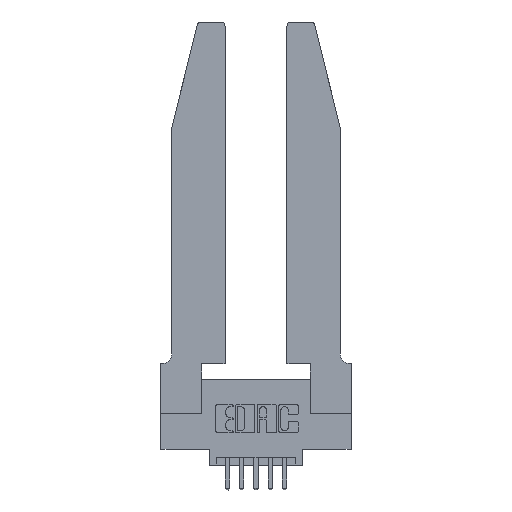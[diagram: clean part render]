
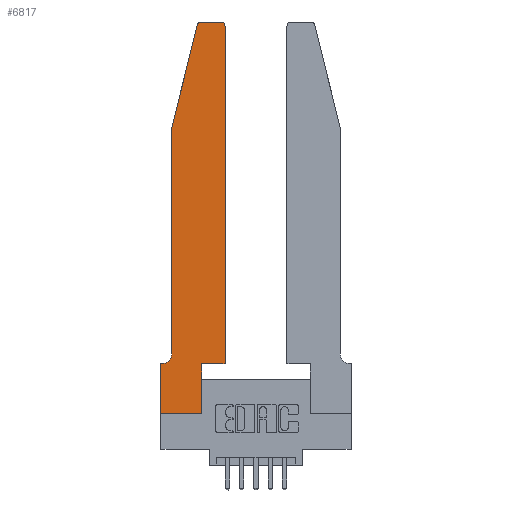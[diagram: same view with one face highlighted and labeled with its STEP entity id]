
A CAD part, top view. The second image highlights one B-rep face of the part: STEP entity #6817.
In plain terms, the highlighted planar face has unit normal (0, 0, 1).
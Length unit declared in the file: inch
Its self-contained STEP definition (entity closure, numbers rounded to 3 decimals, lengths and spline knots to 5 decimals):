
#37 = DIRECTION ( 'NONE',  ( -1., 0., 0. ) ) ;
#279 = CARTESIAN_POINT ( 'NONE',  ( 0., 0., 0.37 ) ) ;
#333 = FACE_OUTER_BOUND ( 'NONE', #13495, .T. ) ;
#451 = CARTESIAN_POINT ( 'NONE',  ( 0.25487, 2.72718, 0.37 ) ) ;
#506 = CIRCLE ( 'NONE', #3302, 0.03 ) ;
#507 = DIRECTION ( 'NONE',  ( 1., 0., 0. ) ) ;
#512 = VECTOR ( 'NONE', #12352, 39.37008 ) ;
#652 = VERTEX_POINT ( 'NONE', #10026 ) ;
#686 = CARTESIAN_POINT ( 'NONE',  ( 0.284, 2.75, 0.37 ) ) ;
#1162 = DIRECTION ( 'NONE',  ( 1., 0., 0. ) ) ;
#1601 = VECTOR ( 'NONE', #37, 39.37008 ) ;
#1735 = CARTESIAN_POINT ( 'NONE',  ( 0.4205, 2.75, 0.37 ) ) ;
#1758 = ORIENTED_EDGE ( 'NONE', *, *, #10402, .T. ) ;
#1817 = CARTESIAN_POINT ( 'NONE',  ( 0., 0.35, 0.37 ) ) ;
#2242 = VECTOR ( 'NONE', #5406, 39.37008 ) ;
#2355 = EDGE_CURVE ( 'NONE', #13267, #9905, #3625, .T. ) ;
#2409 = LINE ( 'NONE', #9857, #2242 ) ;
#2546 = CARTESIAN_POINT ( 'NONE',  ( 0.4505, 2.72, 0.37 ) ) ;
#2553 = LINE ( 'NONE', #13934, #6417 ) ;
#3101 = VECTOR ( 'NONE', #4909, 39.37008 ) ;
#3121 = CARTESIAN_POINT ( 'NONE',  ( 0.0755, 2., 0.37 ) ) ;
#3213 = CARTESIAN_POINT ( 'NONE',  ( 0.2605, 2.75, 0.37 ) ) ;
#3248 = VECTOR ( 'NONE', #7349, 39.37008 ) ;
#3302 = AXIS2_PLACEMENT_3D ( 'NONE', #6360, #9641, #8470 ) ;
#3325 = VERTEX_POINT ( 'NONE', #3121 ) ;
#3347 = DIRECTION ( 'NONE',  ( 0., 0., -1. ) ) ;
#3625 = CIRCLE ( 'NONE', #7901, 0.03 ) ;
#3635 = CARTESIAN_POINT ( 'NONE',  ( 0.2865, 0.35, 0.37 ) ) ;
#3755 = EDGE_CURVE ( 'NONE', #9957, #4941, #4782, .T. ) ;
#3877 = AXIS2_PLACEMENT_3D ( 'NONE', #4842, #7938, #5832 ) ;
#3881 = EDGE_CURVE ( 'NONE', #652, #9957, #8471, .T. ) ;
#3985 = LINE ( 'NONE', #8696, #4813 ) ;
#4170 = EDGE_CURVE ( 'NONE', #5579, #11973, #2409, .T. ) ;
#4488 = ORIENTED_EDGE ( 'NONE', *, *, #2355, .T. ) ;
#4615 = CARTESIAN_POINT ( 'NONE',  ( 0.0755, 2., 0.37 ) ) ;
#4660 = DIRECTION ( 'NONE',  ( -0.239, -0.971, 0. ) ) ;
#4782 = LINE ( 'NONE', #11767, #1601 ) ;
#4813 = VECTOR ( 'NONE', #1162, 39.37008 ) ;
#4830 = EDGE_CURVE ( 'NONE', #11973, #13267, #2553, .T. ) ;
#4842 = CARTESIAN_POINT ( 'NONE',  ( 0., 0.35, 0.37 ) ) ;
#4868 = LINE ( 'NONE', #3635, #512 ) ;
#4909 = DIRECTION ( 'NONE',  ( 0., -1., 0. ) ) ;
#4941 = VERTEX_POINT ( 'NONE', #1817 ) ;
#5387 = ORIENTED_EDGE ( 'NONE', *, *, #9476, .T. ) ;
#5406 = DIRECTION ( 'NONE',  ( 1., 0., 0. ) ) ;
#5408 = VERTEX_POINT ( 'NONE', #7344 ) ;
#5548 = CARTESIAN_POINT ( 'NONE',  ( 0.0055, 0.42, 0.37 ) ) ;
#5579 = VERTEX_POINT ( 'NONE', #13900 ) ;
#5659 = DIRECTION ( 'NONE',  ( -1., 0., 0. ) ) ;
#5832 = DIRECTION ( 'NONE',  ( 1., 0., 0. ) ) ;
#6146 = EDGE_CURVE ( 'NONE', #9905, #7798, #9243, .T. ) ;
#6307 = ORIENTED_EDGE ( 'NONE', *, *, #4170, .T. ) ;
#6360 = CARTESIAN_POINT ( 'NONE',  ( 0.284, 2.72, 0.37 ) ) ;
#6417 = VECTOR ( 'NONE', #10782, 39.37008 ) ;
#6817 = ADVANCED_FACE ( 'NONE', ( #333 ), #6868, .T. ) ;
#6849 = EDGE_CURVE ( 'NONE', #7588, #5579, #4868, .T. ) ;
#6868 = PLANE ( 'NONE',  #3877 ) ;
#7344 = CARTESIAN_POINT ( 'NONE',  ( 0., 0., 0.37 ) ) ;
#7349 = DIRECTION ( 'NONE',  ( 0., -1., 0. ) ) ;
#7588 = VERTEX_POINT ( 'NONE', #7680 ) ;
#7680 = CARTESIAN_POINT ( 'NONE',  ( 0.2865, 0., 0.37 ) ) ;
#7757 = DIRECTION ( 'NONE',  ( -1., 0., 0. ) ) ;
#7792 = LINE ( 'NONE', #279, #3101 ) ;
#7798 = VERTEX_POINT ( 'NONE', #686 ) ;
#7901 = AXIS2_PLACEMENT_3D ( 'NONE', #13261, #8991, #507 ) ;
#7938 = DIRECTION ( 'NONE',  ( 0., 0., 1. ) ) ;
#8226 = VECTOR ( 'NONE', #5659, 39.37008 ) ;
#8354 = CARTESIAN_POINT ( 'NONE',  ( 0.0755, 2., 0.37 ) ) ;
#8466 = EDGE_CURVE ( 'NONE', #10923, #3325, #11374, .T. ) ;
#8470 = DIRECTION ( 'NONE',  ( 1., 0., 0. ) ) ;
#8471 = CIRCLE ( 'NONE', #11391, 0.07 ) ;
#8679 = EDGE_CURVE ( 'NONE', #5408, #7588, #3985, .T. ) ;
#8696 = CARTESIAN_POINT ( 'NONE',  ( 0., 0., 0.37 ) ) ;
#8845 = ORIENTED_EDGE ( 'NONE', *, *, #8679, .T. ) ;
#8906 = CARTESIAN_POINT ( 'NONE',  ( 0.4505, 0.35, 0.37 ) ) ;
#8991 = DIRECTION ( 'NONE',  ( 0., 0., 1. ) ) ;
#9243 = LINE ( 'NONE', #3213, #8226 ) ;
#9279 = ORIENTED_EDGE ( 'NONE', *, *, #3755, .T. ) ;
#9476 = EDGE_CURVE ( 'NONE', #3325, #652, #12816, .T. ) ;
#9641 = DIRECTION ( 'NONE',  ( 0., 0., 1. ) ) ;
#9752 = ORIENTED_EDGE ( 'NONE', *, *, #6849, .T. ) ;
#9857 = CARTESIAN_POINT ( 'NONE',  ( 0.4505, 0.35, 0.37 ) ) ;
#9905 = VERTEX_POINT ( 'NONE', #1735 ) ;
#9957 = VERTEX_POINT ( 'NONE', #11400 ) ;
#10026 = CARTESIAN_POINT ( 'NONE',  ( 0.0755, 0.42, 0.37 ) ) ;
#10352 = ORIENTED_EDGE ( 'NONE', *, *, #8466, .T. ) ;
#10402 = EDGE_CURVE ( 'NONE', #4941, #5408, #7792, .T. ) ;
#10611 = ORIENTED_EDGE ( 'NONE', *, *, #13032, .T. ) ;
#10782 = DIRECTION ( 'NONE',  ( 0., 1., 0. ) ) ;
#10923 = VERTEX_POINT ( 'NONE', #451 ) ;
#11240 = ORIENTED_EDGE ( 'NONE', *, *, #4830, .T. ) ;
#11374 = LINE ( 'NONE', #4615, #13746 ) ;
#11391 = AXIS2_PLACEMENT_3D ( 'NONE', #5548, #3347, #7757 ) ;
#11400 = CARTESIAN_POINT ( 'NONE',  ( 0.0055, 0.35, 0.37 ) ) ;
#11767 = CARTESIAN_POINT ( 'NONE',  ( 0.0755, 0.35, 0.37 ) ) ;
#11973 = VERTEX_POINT ( 'NONE', #8906 ) ;
#12233 = ORIENTED_EDGE ( 'NONE', *, *, #6146, .T. ) ;
#12352 = DIRECTION ( 'NONE',  ( 0., 1., 0. ) ) ;
#12816 = LINE ( 'NONE', #8354, #3248 ) ;
#12910 = ORIENTED_EDGE ( 'NONE', *, *, #3881, .T. ) ;
#13032 = EDGE_CURVE ( 'NONE', #7798, #10923, #506, .T. ) ;
#13261 = CARTESIAN_POINT ( 'NONE',  ( 0.4205, 2.72, 0.37 ) ) ;
#13267 = VERTEX_POINT ( 'NONE', #2546 ) ;
#13495 = EDGE_LOOP ( 'NONE', ( #12233, #10611, #10352, #5387, #12910, #9279, #1758, #8845, #9752, #6307, #11240, #4488 ) ) ;
#13746 = VECTOR ( 'NONE', #4660, 39.37008 ) ;
#13900 = CARTESIAN_POINT ( 'NONE',  ( 0.2865, 0.35, 0.37 ) ) ;
#13934 = CARTESIAN_POINT ( 'NONE',  ( 0.4505, 0.35, 0.37 ) ) ;
